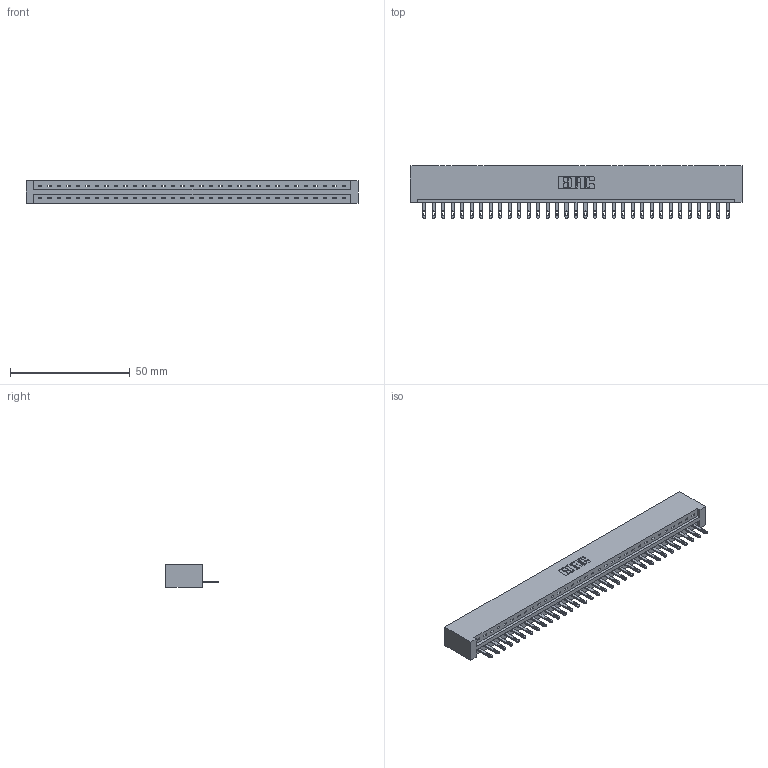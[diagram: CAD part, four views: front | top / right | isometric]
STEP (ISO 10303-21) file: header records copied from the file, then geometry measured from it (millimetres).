
FILE_DESCRIPTION (( 'STEP AP203' ), '1' );
FILE_NAME ('887-033-500-101.STEP', '2020-09-20T21:21:00', ( '' ), ( '' ), 'SwSTEP 2.0', 'SolidWorks 2020', '' );
FILE_SCHEMA (( 'CONFIG_CONTROL_DESIGN' ));
Length unit declared in the file: inch
Products named in the file (3): 837 Part_No Mounting Lugs; 345-292-001_345-293-100; 887-033-500-101
Assembly tree (34 placements, depth 2):
  887-033-500-101
    837 Part_No Mounting Lugs
    345-292-001_345-293-100  x33
Bounding box: 138.63 x 21.85 x 9.4 mm (x, y, z)
Volume: 15055.1 mm3; surface area: 15565.8 mm2
Topology: 34 solids, 34 shells, 2020 faces, 6227 edges, 4150 vertices
Faces by surface type: plane 1386, cylinder 634
Entity records: 25347 total; most frequent: CARTESIAN_POINT 4421, ORIENTED_EDGE 4390, DIRECTION 3733, EDGE_CURVE 2195, LINE 2071, VECTOR 2071, VERTEX_POINT 1462, AXIS2_PLACEMENT_3D 831
